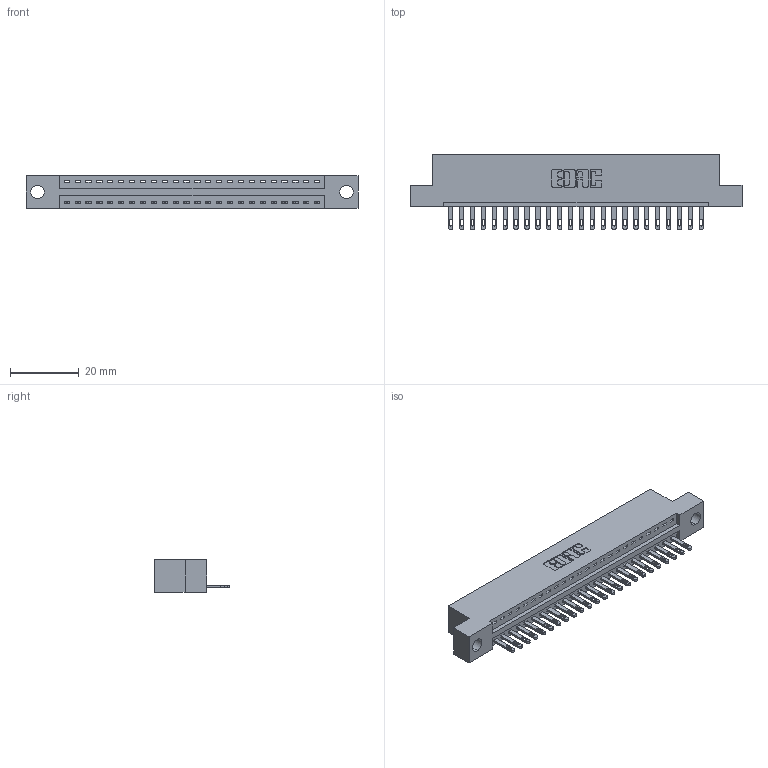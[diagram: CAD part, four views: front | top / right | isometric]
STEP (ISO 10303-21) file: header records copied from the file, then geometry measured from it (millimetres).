
FILE_DESCRIPTION (( 'STEP AP203' ), '1' );
FILE_NAME ('346-024-500-104.STEP', '2022-05-05T22:07:04', ( '' ), ( '' ), 'SwSTEP 2.0', 'SolidWorks 2020', '' );
FILE_SCHEMA (( 'CONFIG_CONTROL_DESIGN' ));
Length unit declared in the file: inch
Products named in the file (3): 346-024-500-104; 346 Part_Flush Mounting Lugs - 0.156 Dia-TH; 345-292-001_345-293-100
Assembly tree (25 placements, depth 2):
  346-024-500-104
    346 Part_Flush Mounting Lugs - 0.156 Dia-TH
    345-292-001_345-293-100  x24
Bounding box: 96.77 x 21.84 x 9.4 mm (x, y, z)
Volume: 9048.3 mm3; surface area: 11008.1 mm2
Topology: 25 solids, 25 shells, 1432 faces, 4397 edges, 2930 vertices
Faces by surface type: plane 906, cylinder 526
Entity records: 17667 total; most frequent: CARTESIAN_POINT 3042, ORIENTED_EDGE 2998, DIRECTION 2707, EDGE_CURVE 1499, VECTOR 1267, LINE 1267, VERTEX_POINT 998, AXIS2_PLACEMENT_3D 720
